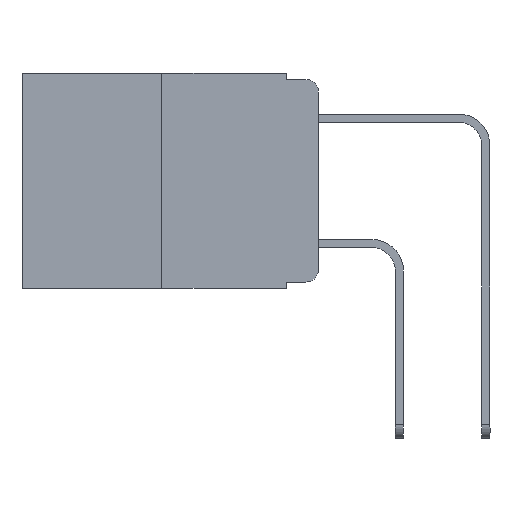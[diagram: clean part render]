
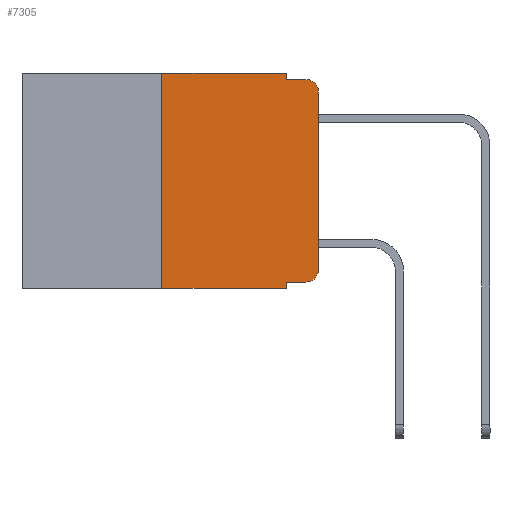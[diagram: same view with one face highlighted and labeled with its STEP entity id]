
A CAD part, left-side view. The second image highlights one B-rep face of the part: STEP entity #7305.
In plain terms, the highlighted planar face has unit normal (-1, 0, 0).
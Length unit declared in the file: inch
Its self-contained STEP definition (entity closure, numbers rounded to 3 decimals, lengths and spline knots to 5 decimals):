
#283 = DIRECTION ( 'NONE',  ( 0., 0., -1. ) ) ;
#426 = CARTESIAN_POINT ( 'NONE',  ( 0., 0.25, 0. ) ) ;
#769 = CARTESIAN_POINT ( 'NONE',  ( 0., 0.051, -0.01 ) ) ;
#821 = VERTEX_POINT ( 'NONE', #1472 ) ;
#844 = DIRECTION ( 'NONE',  ( 0., -1., 0. ) ) ;
#907 = ORIENTED_EDGE ( 'NONE', *, *, #14180, .F. ) ;
#1231 = ORIENTED_EDGE ( 'NONE', *, *, #15084, .F. ) ;
#1472 = CARTESIAN_POINT ( 'NONE',  ( 0., 0.02, -0.01 ) ) ;
#1779 = VECTOR ( 'NONE', #283, 39.37008 ) ;
#1852 = CARTESIAN_POINT ( 'NONE',  ( 0., 0.051, 0. ) ) ;
#2510 = CARTESIAN_POINT ( 'NONE',  ( 0., 0.25, -0.343 ) ) ;
#2524 = EDGE_LOOP ( 'NONE', ( #9405, #15934, #907, #18732, #1231, #17211, #6086, #11112, #20462, #16936 ) ) ;
#2725 = EDGE_CURVE ( 'NONE', #3372, #20987, #24126, .T. ) ;
#2821 = VERTEX_POINT ( 'NONE', #14939 ) ;
#2941 = DIRECTION ( 'NONE',  ( 0., 0., -1. ) ) ;
#3372 = VERTEX_POINT ( 'NONE', #2510 ) ;
#4418 = LINE ( 'NONE', #12773, #20311 ) ;
#4706 = EDGE_CURVE ( 'NONE', #15662, #2821, #4418, .T. ) ;
#4731 = PLANE ( 'NONE',  #13915 ) ;
#5313 = DIRECTION ( 'NONE',  ( 0., 0., -1. ) ) ;
#5786 = LINE ( 'NONE', #14149, #12979 ) ;
#5876 = EDGE_CURVE ( 'NONE', #3372, #6896, #5786, .T. ) ;
#6086 = ORIENTED_EDGE ( 'NONE', *, *, #2725, .T. ) ;
#6453 = CARTESIAN_POINT ( 'NONE',  ( 0., 0.051, -0.333 ) ) ;
#6522 = LINE ( 'NONE', #15022, #1779 ) ;
#6896 = VERTEX_POINT ( 'NONE', #426 ) ;
#7055 = VECTOR ( 'NONE', #844, 39.37008 ) ;
#7122 = DIRECTION ( 'NONE',  ( 0., -1., 0. ) ) ;
#7183 = EDGE_CURVE ( 'NONE', #13943, #20987, #16768, .T. ) ;
#7305 = ADVANCED_FACE ( 'NONE', ( #15271 ), #4731, .F. ) ;
#7583 = EDGE_CURVE ( 'NONE', #13943, #16986, #18776, .T. ) ;
#8237 = VECTOR ( 'NONE', #14825, 39.37008 ) ;
#8594 = CARTESIAN_POINT ( 'NONE',  ( 0., 0.051, -0.333 ) ) ;
#8871 = VERTEX_POINT ( 'NONE', #1852 ) ;
#9405 = ORIENTED_EDGE ( 'NONE', *, *, #4706, .T. ) ;
#9606 = CIRCLE ( 'NONE', #15742, 0.02 ) ;
#10909 = EDGE_CURVE ( 'NONE', #2821, #821, #9606, .T. ) ;
#11112 = ORIENTED_EDGE ( 'NONE', *, *, #7183, .F. ) ;
#11246 = EDGE_CURVE ( 'NONE', #8871, #11764, #6522, .T. ) ;
#11638 = LINE ( 'NONE', #13568, #19023 ) ;
#11764 = VERTEX_POINT ( 'NONE', #769 ) ;
#12414 = AXIS2_PLACEMENT_3D ( 'NONE', #18524, #18384, #24122 ) ;
#12676 = CARTESIAN_POINT ( 'NONE',  ( 0., 0.051, 0. ) ) ;
#12773 = CARTESIAN_POINT ( 'NONE',  ( 0., 0., 0. ) ) ;
#12814 = DIRECTION ( 'NONE',  ( 0., 0., -1. ) ) ;
#12979 = VECTOR ( 'NONE', #20417, 39.37008 ) ;
#13088 = CARTESIAN_POINT ( 'NONE',  ( 0., 0.473, 0. ) ) ;
#13568 = CARTESIAN_POINT ( 'NONE',  ( 0., 0.473, 0. ) ) ;
#13915 = AXIS2_PLACEMENT_3D ( 'NONE', #13088, #19501, #12814 ) ;
#13943 = VERTEX_POINT ( 'NONE', #8594 ) ;
#14149 = CARTESIAN_POINT ( 'NONE',  ( 0., 0.25, 0. ) ) ;
#14180 = EDGE_CURVE ( 'NONE', #11764, #821, #15847, .T. ) ;
#14825 = DIRECTION ( 'NONE',  ( 0., -1., 0. ) ) ;
#14939 = CARTESIAN_POINT ( 'NONE',  ( 0., 0., -0.03 ) ) ;
#15022 = CARTESIAN_POINT ( 'NONE',  ( 0., 0.051, 0. ) ) ;
#15084 = EDGE_CURVE ( 'NONE', #6896, #8871, #11638, .T. ) ;
#15271 = FACE_OUTER_BOUND ( 'NONE', #2524, .T. ) ;
#15662 = VERTEX_POINT ( 'NONE', #20605 ) ;
#15742 = AXIS2_PLACEMENT_3D ( 'NONE', #17892, #22135, #5313 ) ;
#15847 = LINE ( 'NONE', #21572, #7055 ) ;
#15934 = ORIENTED_EDGE ( 'NONE', *, *, #10909, .T. ) ;
#16525 = VECTOR ( 'NONE', #2941, 39.37008 ) ;
#16768 = LINE ( 'NONE', #12676, #16525 ) ;
#16936 = ORIENTED_EDGE ( 'NONE', *, *, #26946, .T. ) ;
#16986 = VERTEX_POINT ( 'NONE', #26026 ) ;
#17211 = ORIENTED_EDGE ( 'NONE', *, *, #5876, .F. ) ;
#17711 = CARTESIAN_POINT ( 'NONE',  ( 0., 0.473, -0.343 ) ) ;
#17892 = CARTESIAN_POINT ( 'NONE',  ( 0., 0.02, -0.03 ) ) ;
#18384 = DIRECTION ( 'NONE',  ( -1., 0., 0. ) ) ;
#18524 = CARTESIAN_POINT ( 'NONE',  ( 0., 0.02, -0.313 ) ) ;
#18732 = ORIENTED_EDGE ( 'NONE', *, *, #11246, .F. ) ;
#18776 = LINE ( 'NONE', #6453, #8237 ) ;
#19023 = VECTOR ( 'NONE', #7122, 39.37008 ) ;
#19497 = CARTESIAN_POINT ( 'NONE',  ( 0., 0.051, -0.343 ) ) ;
#19501 = DIRECTION ( 'NONE',  ( 1., 0., 0. ) ) ;
#19680 = VECTOR ( 'NONE', #21949, 39.37008 ) ;
#19820 = CIRCLE ( 'NONE', #12414, 0.02 ) ;
#20311 = VECTOR ( 'NONE', #21094, 39.37008 ) ;
#20417 = DIRECTION ( 'NONE',  ( 0., 0., 1. ) ) ;
#20462 = ORIENTED_EDGE ( 'NONE', *, *, #7583, .T. ) ;
#20605 = CARTESIAN_POINT ( 'NONE',  ( 0., 0., -0.313 ) ) ;
#20987 = VERTEX_POINT ( 'NONE', #19497 ) ;
#21094 = DIRECTION ( 'NONE',  ( 0., 0., 1. ) ) ;
#21572 = CARTESIAN_POINT ( 'NONE',  ( 0., 0.051, -0.01 ) ) ;
#21949 = DIRECTION ( 'NONE',  ( 0., -1., 0. ) ) ;
#22135 = DIRECTION ( 'NONE',  ( -1., 0., 0. ) ) ;
#24122 = DIRECTION ( 'NONE',  ( 0., 0., -1. ) ) ;
#24126 = LINE ( 'NONE', #17711, #19680 ) ;
#26026 = CARTESIAN_POINT ( 'NONE',  ( 0., 0.02, -0.333 ) ) ;
#26946 = EDGE_CURVE ( 'NONE', #16986, #15662, #19820, .T. ) ;
